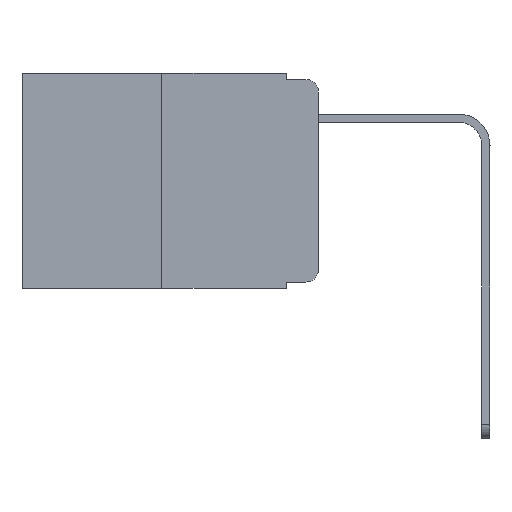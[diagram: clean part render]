
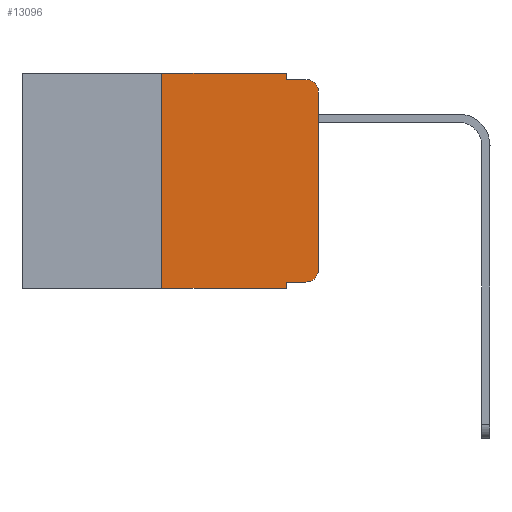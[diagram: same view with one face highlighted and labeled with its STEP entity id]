
A CAD part, left-side view. The second image highlights one B-rep face of the part: STEP entity #13096.
In plain terms, the highlighted planar face has unit normal (-1, 0, 0).
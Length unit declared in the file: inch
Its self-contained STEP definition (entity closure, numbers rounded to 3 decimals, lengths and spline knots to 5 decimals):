
#16 = EDGE_CURVE ( 'NONE', #4778, #362, #4104, .T. ) ;
#282 = VERTEX_POINT ( 'NONE', #14042 ) ;
#332 = AXIS2_PLACEMENT_3D ( 'NONE', #8398, #1562, #12972 ) ;
#344 = ORIENTED_EDGE ( 'NONE', *, *, #12620, .F. ) ;
#362 = VERTEX_POINT ( 'NONE', #7130 ) ;
#676 = DIRECTION ( 'NONE',  ( 0., 0., -1. ) ) ;
#771 = EDGE_CURVE ( 'NONE', #11543, #1627, #4804, .T. ) ;
#1216 = DIRECTION ( 'NONE',  ( 0., -1., 0. ) ) ;
#1386 = CARTESIAN_POINT ( 'NONE',  ( 0., 0.051, -0.343 ) ) ;
#1464 = DIRECTION ( 'NONE',  ( 0., 0., -1. ) ) ;
#1562 = DIRECTION ( 'NONE',  ( -1., 0., 0. ) ) ;
#1627 = VERTEX_POINT ( 'NONE', #7670 ) ;
#1761 = VECTOR ( 'NONE', #12851, 39.37008 ) ;
#1816 = CARTESIAN_POINT ( 'NONE',  ( 0., 0.051, 0. ) ) ;
#1971 = CARTESIAN_POINT ( 'NONE',  ( 0., 0.02, -0.03 ) ) ;
#2059 = CARTESIAN_POINT ( 'NONE',  ( 0., 0., -0.313 ) ) ;
#2114 = ORIENTED_EDGE ( 'NONE', *, *, #7210, .F. ) ;
#2137 = EDGE_CURVE ( 'NONE', #5120, #12861, #14175, .T. ) ;
#2310 = DIRECTION ( 'NONE',  ( 1., 0., 0. ) ) ;
#2419 = EDGE_CURVE ( 'NONE', #1627, #14475, #6513, .T. ) ;
#2660 = EDGE_CURVE ( 'NONE', #282, #12861, #13822, .T. ) ;
#3216 = ORIENTED_EDGE ( 'NONE', *, *, #7674, .T. ) ;
#3349 = CARTESIAN_POINT ( 'NONE',  ( 0., 0., 0. ) ) ;
#3665 = CARTESIAN_POINT ( 'NONE',  ( 0., 0.051, 0. ) ) ;
#4104 = LINE ( 'NONE', #7093, #9794 ) ;
#4542 = EDGE_LOOP ( 'NONE', ( #3216, #10420, #7926, #344, #2114, #9277, #9572, #13489, #6548, #6982 ) ) ;
#4778 = VERTEX_POINT ( 'NONE', #6931 ) ;
#4786 = VECTOR ( 'NONE', #10820, 39.37008 ) ;
#4804 = LINE ( 'NONE', #4849, #1761 ) ;
#4846 = CARTESIAN_POINT ( 'NONE',  ( 0., 0.051, -0.333 ) ) ;
#4849 = CARTESIAN_POINT ( 'NONE',  ( 0., 0.051, -0.333 ) ) ;
#5120 = VERTEX_POINT ( 'NONE', #11055 ) ;
#5150 = CARTESIAN_POINT ( 'NONE',  ( 0., 0.473, 0. ) ) ;
#5174 = AXIS2_PLACEMENT_3D ( 'NONE', #12004, #2310, #8306 ) ;
#5238 = VECTOR ( 'NONE', #7704, 39.37008 ) ;
#6513 = CIRCLE ( 'NONE', #332, 0.02 ) ;
#6548 = ORIENTED_EDGE ( 'NONE', *, *, #771, .T. ) ;
#6931 = CARTESIAN_POINT ( 'NONE',  ( 0., 0.25, -0.343 ) ) ;
#6982 = ORIENTED_EDGE ( 'NONE', *, *, #2419, .T. ) ;
#7093 = CARTESIAN_POINT ( 'NONE',  ( 0., 0.25, 0. ) ) ;
#7130 = CARTESIAN_POINT ( 'NONE',  ( 0., 0.25, 0. ) ) ;
#7187 = DIRECTION ( 'NONE',  ( 0., 0., 1. ) ) ;
#7210 = EDGE_CURVE ( 'NONE', #362, #14217, #12119, .T. ) ;
#7284 = LINE ( 'NONE', #3349, #9026 ) ;
#7500 = DIRECTION ( 'NONE',  ( 0., -1., 0. ) ) ;
#7670 = CARTESIAN_POINT ( 'NONE',  ( 0., 0.02, -0.333 ) ) ;
#7674 = EDGE_CURVE ( 'NONE', #14475, #5120, #7284, .T. ) ;
#7704 = DIRECTION ( 'NONE',  ( 0., -1., 0. ) ) ;
#7906 = VECTOR ( 'NONE', #1216, 39.37008 ) ;
#7926 = ORIENTED_EDGE ( 'NONE', *, *, #2660, .F. ) ;
#8074 = LINE ( 'NONE', #3665, #12023 ) ;
#8306 = DIRECTION ( 'NONE',  ( 0., 0., -1. ) ) ;
#8398 = CARTESIAN_POINT ( 'NONE',  ( 0., 0.02, -0.313 ) ) ;
#9026 = VECTOR ( 'NONE', #13634, 39.37008 ) ;
#9260 = EDGE_CURVE ( 'NONE', #4778, #12304, #13648, .T. ) ;
#9277 = ORIENTED_EDGE ( 'NONE', *, *, #16, .F. ) ;
#9385 = FACE_OUTER_BOUND ( 'NONE', #4542, .T. ) ;
#9572 = ORIENTED_EDGE ( 'NONE', *, *, #9260, .T. ) ;
#9794 = VECTOR ( 'NONE', #7187, 39.37008 ) ;
#9838 = EDGE_CURVE ( 'NONE', #11543, #12304, #8074, .T. ) ;
#10420 = ORIENTED_EDGE ( 'NONE', *, *, #2137, .T. ) ;
#10652 = LINE ( 'NONE', #10967, #4786 ) ;
#10820 = DIRECTION ( 'NONE',  ( 0., 0., -1. ) ) ;
#10967 = CARTESIAN_POINT ( 'NONE',  ( 0., 0.051, 0. ) ) ;
#11028 = VECTOR ( 'NONE', #7500, 39.37008 ) ;
#11055 = CARTESIAN_POINT ( 'NONE',  ( 0., 0., -0.03 ) ) ;
#11543 = VERTEX_POINT ( 'NONE', #4846 ) ;
#11826 = CARTESIAN_POINT ( 'NONE',  ( 0., 0.02, -0.01 ) ) ;
#12004 = CARTESIAN_POINT ( 'NONE',  ( 0., 0.473, 0. ) ) ;
#12023 = VECTOR ( 'NONE', #1464, 39.37008 ) ;
#12111 = AXIS2_PLACEMENT_3D ( 'NONE', #1971, #14535, #676 ) ;
#12119 = LINE ( 'NONE', #5150, #11028 ) ;
#12304 = VERTEX_POINT ( 'NONE', #1386 ) ;
#12340 = CARTESIAN_POINT ( 'NONE',  ( 0., 0.473, -0.343 ) ) ;
#12620 = EDGE_CURVE ( 'NONE', #14217, #282, #10652, .T. ) ;
#12851 = DIRECTION ( 'NONE',  ( 0., -1., 0. ) ) ;
#12861 = VERTEX_POINT ( 'NONE', #11826 ) ;
#12972 = DIRECTION ( 'NONE',  ( 0., 0., -1. ) ) ;
#13096 = ADVANCED_FACE ( 'NONE', ( #9385 ), #13958, .F. ) ;
#13489 = ORIENTED_EDGE ( 'NONE', *, *, #9838, .F. ) ;
#13634 = DIRECTION ( 'NONE',  ( 0., 0., 1. ) ) ;
#13648 = LINE ( 'NONE', #12340, #7906 ) ;
#13822 = LINE ( 'NONE', #14296, #5238 ) ;
#13958 = PLANE ( 'NONE',  #5174 ) ;
#14042 = CARTESIAN_POINT ( 'NONE',  ( 0., 0.051, -0.01 ) ) ;
#14175 = CIRCLE ( 'NONE', #12111, 0.02 ) ;
#14217 = VERTEX_POINT ( 'NONE', #1816 ) ;
#14296 = CARTESIAN_POINT ( 'NONE',  ( 0., 0.051, -0.01 ) ) ;
#14475 = VERTEX_POINT ( 'NONE', #2059 ) ;
#14535 = DIRECTION ( 'NONE',  ( -1., 0., 0. ) ) ;
